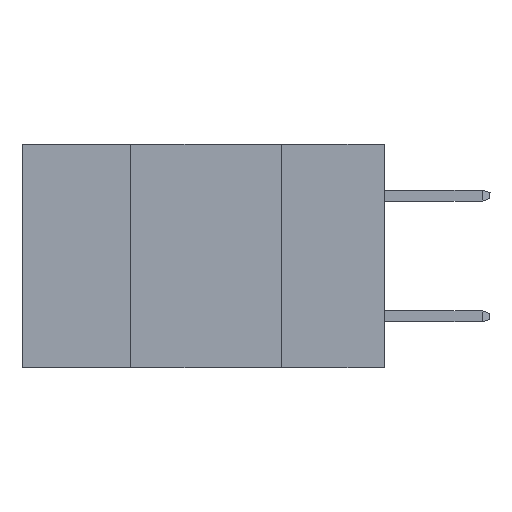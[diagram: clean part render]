
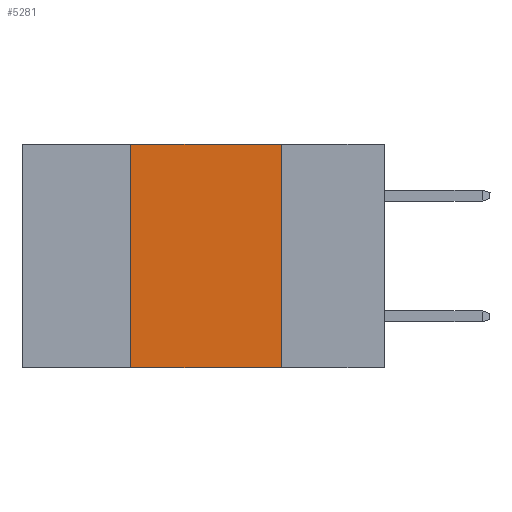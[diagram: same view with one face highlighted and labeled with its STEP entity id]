
A CAD part, left-side view. The second image highlights one B-rep face of the part: STEP entity #5281.
In plain terms, the highlighted planar face has unit normal (-1, 0, 0).
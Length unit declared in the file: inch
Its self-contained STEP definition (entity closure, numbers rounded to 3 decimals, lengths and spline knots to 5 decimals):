
#45 = VERTEX_POINT ( 'NONE', #2608 ) ;
#267 = VECTOR ( 'NONE', #2988, 39.37008 ) ;
#960 = LINE ( 'NONE', #15198, #9388 ) ;
#2608 = CARTESIAN_POINT ( 'NONE',  ( 0., 0.17, 0. ) ) ;
#2988 = DIRECTION ( 'NONE',  ( 0., 0., 1. ) ) ;
#3046 = DIRECTION ( 'NONE',  ( 0., -1., 0. ) ) ;
#3133 = PLANE ( 'NONE',  #11890 ) ;
#3726 = ORIENTED_EDGE ( 'NONE', *, *, #15168, .F. ) ;
#4201 = ORIENTED_EDGE ( 'NONE', *, *, #14257, .F. ) ;
#5221 = DIRECTION ( 'NONE',  ( 0., -1., 0. ) ) ;
#5281 = ADVANCED_FACE ( 'NONE', ( #15538 ), #3133, .F. ) ;
#6162 = CARTESIAN_POINT ( 'NONE',  ( 0., 0.6, 0. ) ) ;
#7321 = VECTOR ( 'NONE', #3046, 39.37008 ) ;
#7491 = EDGE_CURVE ( 'NONE', #10245, #45, #11571, .T. ) ;
#7652 = DIRECTION ( 'NONE',  ( 0., 0., -1. ) ) ;
#8699 = VERTEX_POINT ( 'NONE', #17452 ) ;
#9363 = VERTEX_POINT ( 'NONE', #14801 ) ;
#9388 = VECTOR ( 'NONE', #5221, 39.37008 ) ;
#10245 = VERTEX_POINT ( 'NONE', #16140 ) ;
#10271 = VECTOR ( 'NONE', #12066, 39.37008 ) ;
#10625 = CARTESIAN_POINT ( 'NONE',  ( 0., 0.17, 0. ) ) ;
#11506 = ORIENTED_EDGE ( 'NONE', *, *, #7491, .F. ) ;
#11571 = LINE ( 'NONE', #13227, #7321 ) ;
#11890 = AXIS2_PLACEMENT_3D ( 'NONE', #6162, #16066, #7652 ) ;
#11968 = ORIENTED_EDGE ( 'NONE', *, *, #13308, .T. ) ;
#12065 = LINE ( 'NONE', #13169, #267 ) ;
#12066 = DIRECTION ( 'NONE',  ( 0., 0., -1. ) ) ;
#13169 = CARTESIAN_POINT ( 'NONE',  ( 0., 0.42, 0. ) ) ;
#13227 = CARTESIAN_POINT ( 'NONE',  ( 0., 0.6, 0. ) ) ;
#13308 = EDGE_CURVE ( 'NONE', #9363, #8699, #960, .T. ) ;
#14017 = LINE ( 'NONE', #10625, #10271 ) ;
#14257 = EDGE_CURVE ( 'NONE', #9363, #10245, #12065, .T. ) ;
#14793 = EDGE_LOOP ( 'NONE', ( #3726, #11506, #4201, #11968 ) ) ;
#14801 = CARTESIAN_POINT ( 'NONE',  ( 0., 0.42, -0.37 ) ) ;
#15168 = EDGE_CURVE ( 'NONE', #45, #8699, #14017, .T. ) ;
#15198 = CARTESIAN_POINT ( 'NONE',  ( 0., 0.6, -0.37 ) ) ;
#15538 = FACE_OUTER_BOUND ( 'NONE', #14793, .T. ) ;
#16066 = DIRECTION ( 'NONE',  ( 1., 0., 0. ) ) ;
#16140 = CARTESIAN_POINT ( 'NONE',  ( 0., 0.42, 0. ) ) ;
#17452 = CARTESIAN_POINT ( 'NONE',  ( 0., 0.17, -0.37 ) ) ;
